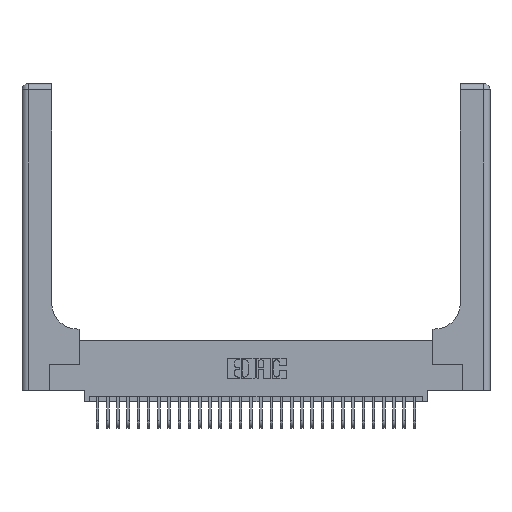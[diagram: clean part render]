
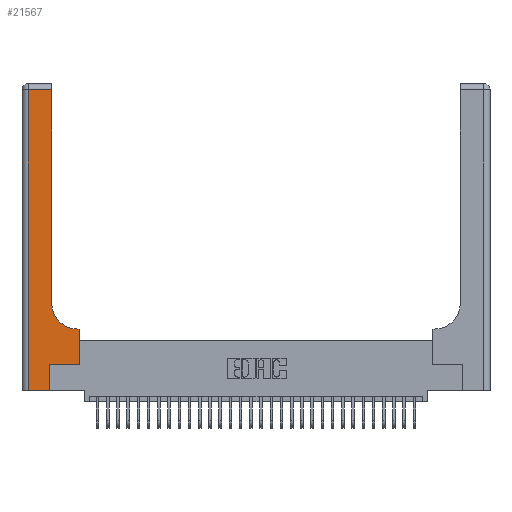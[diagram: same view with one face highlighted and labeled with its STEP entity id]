
A CAD part, top view. The second image highlights one B-rep face of the part: STEP entity #21567.
In plain terms, the highlighted planar face has unit normal (0, 0, 1).
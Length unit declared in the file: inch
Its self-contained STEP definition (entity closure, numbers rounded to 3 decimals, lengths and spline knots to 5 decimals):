
#291 = ORIENTED_EDGE ( 'NONE', *, *, #17191, .T. ) ;
#525 = CARTESIAN_POINT ( 'NONE',  ( 0.5585, 0.25, 0.37 ) ) ;
#1414 = FACE_OUTER_BOUND ( 'NONE', #19779, .T. ) ;
#1512 = CARTESIAN_POINT ( 'NONE',  ( 0.269, 0.25, 0.37 ) ) ;
#2704 = CARTESIAN_POINT ( 'NONE',  ( 0.5585, 0.6, 0.37 ) ) ;
#3283 = LINE ( 'NONE', #10654, #8548 ) ;
#3613 = EDGE_CURVE ( 'NONE', #7267, #27339, #28701, .T. ) ;
#3993 = DIRECTION ( 'NONE',  ( -1., 0., 0. ) ) ;
#4004 = DIRECTION ( 'NONE',  ( 0., 1., 0. ) ) ;
#4543 = LINE ( 'NONE', #29493, #17528 ) ;
#4869 = CARTESIAN_POINT ( 'NONE',  ( 0.5415, 0.85, 0.37 ) ) ;
#5541 = VERTEX_POINT ( 'NONE', #20499 ) ;
#6205 = LINE ( 'NONE', #25804, #32009 ) ;
#7267 = VERTEX_POINT ( 'NONE', #17939 ) ;
#7470 = DIRECTION ( 'NONE',  ( 1., 0., 0. ) ) ;
#7866 = CARTESIAN_POINT ( 'NONE',  ( 0.06, 2.94, 0.37 ) ) ;
#8024 = PLANE ( 'NONE',  #22975 ) ;
#8548 = VECTOR ( 'NONE', #33169, 39.37008 ) ;
#8583 = VERTEX_POINT ( 'NONE', #23969 ) ;
#9338 = VERTEX_POINT ( 'NONE', #1512 ) ;
#9535 = LINE ( 'NONE', #29439, #30106 ) ;
#10598 = CIRCLE ( 'NONE', #12292, 0.25 ) ;
#10619 = CARTESIAN_POINT ( 'NONE',  ( 0., 3., 0.37 ) ) ;
#10654 = CARTESIAN_POINT ( 'NONE',  ( 0.269, 0., 0.37 ) ) ;
#12292 = AXIS2_PLACEMENT_3D ( 'NONE', #4869, #22955, #7470 ) ;
#12900 = DIRECTION ( 'NONE',  ( 0., -1., 0. ) ) ;
#13208 = VERTEX_POINT ( 'NONE', #7866 ) ;
#13221 = DIRECTION ( 'NONE',  ( -1., 0., 0. ) ) ;
#13995 = DIRECTION ( 'NONE',  ( 1., 0., 0. ) ) ;
#14160 = CARTESIAN_POINT ( 'NONE',  ( 0.5415, 0.6, 0.37 ) ) ;
#14163 = VECTOR ( 'NONE', #4004, 39.37008 ) ;
#14220 = CARTESIAN_POINT ( 'NONE',  ( 0.269, 0.25, 0.37 ) ) ;
#14276 = LINE ( 'NONE', #525, #28006 ) ;
#14910 = LINE ( 'NONE', #19503, #27798 ) ;
#17191 = EDGE_CURVE ( 'NONE', #9338, #5541, #29421, .T. ) ;
#17528 = VECTOR ( 'NONE', #32068, 39.37008 ) ;
#17809 = ORIENTED_EDGE ( 'NONE', *, *, #25847, .T. ) ;
#17835 = VERTEX_POINT ( 'NONE', #30077 ) ;
#17939 = CARTESIAN_POINT ( 'NONE',  ( 0.2915, 0.85, 0.37 ) ) ;
#19503 = CARTESIAN_POINT ( 'NONE',  ( 0., 2.94, 0.37 ) ) ;
#19715 = ORIENTED_EDGE ( 'NONE', *, *, #24186, .T. ) ;
#19779 = EDGE_LOOP ( 'NONE', ( #20834, #30894, #25755, #32157, #19715, #291, #21763, #31819, #17809 ) ) ;
#20499 = CARTESIAN_POINT ( 'NONE',  ( 0.5585, 0.25, 0.37 ) ) ;
#20834 = ORIENTED_EDGE ( 'NONE', *, *, #3613, .T. ) ;
#21060 = VERTEX_POINT ( 'NONE', #2704 ) ;
#21232 = DIRECTION ( 'NONE',  ( 0., 1., 0. ) ) ;
#21567 = ADVANCED_FACE ( 'NONE', ( #1414 ), #8024, .F. ) ;
#21763 = ORIENTED_EDGE ( 'NONE', *, *, #31767, .T. ) ;
#21778 = EDGE_CURVE ( 'NONE', #17835, #8583, #9535, .T. ) ;
#21905 = DIRECTION ( 'NONE',  ( 1., 0., 0. ) ) ;
#22585 = VECTOR ( 'NONE', #21905, 39.37008 ) ;
#22955 = DIRECTION ( 'NONE',  ( 0., 0., -1. ) ) ;
#22975 = AXIS2_PLACEMENT_3D ( 'NONE', #10619, #28673, #13221 ) ;
#23845 = EDGE_CURVE ( 'NONE', #21060, #31265, #4543, .T. ) ;
#23969 = CARTESIAN_POINT ( 'NONE',  ( 0.269, 0., 0.37 ) ) ;
#24116 = CARTESIAN_POINT ( 'NONE',  ( 0.2915, 2.94, 0.37 ) ) ;
#24186 = EDGE_CURVE ( 'NONE', #8583, #9338, #3283, .T. ) ;
#25755 = ORIENTED_EDGE ( 'NONE', *, *, #31593, .T. ) ;
#25804 = CARTESIAN_POINT ( 'NONE',  ( 0.06, 3., 0.37 ) ) ;
#25847 = EDGE_CURVE ( 'NONE', #31265, #7267, #10598, .T. ) ;
#27339 = VERTEX_POINT ( 'NONE', #24116 ) ;
#27798 = VECTOR ( 'NONE', #3993, 39.37008 ) ;
#28006 = VECTOR ( 'NONE', #21232, 39.37008 ) ;
#28194 = EDGE_CURVE ( 'NONE', #27339, #13208, #14910, .T. ) ;
#28673 = DIRECTION ( 'NONE',  ( 0., 0., -1. ) ) ;
#28701 = LINE ( 'NONE', #32318, #14163 ) ;
#29421 = LINE ( 'NONE', #14220, #22585 ) ;
#29439 = CARTESIAN_POINT ( 'NONE',  ( 0., 0., 0.37 ) ) ;
#29493 = CARTESIAN_POINT ( 'NONE',  ( 0.2915, 0.6, 0.37 ) ) ;
#30077 = CARTESIAN_POINT ( 'NONE',  ( 0.06, 0., 0.37 ) ) ;
#30106 = VECTOR ( 'NONE', #13995, 39.37008 ) ;
#30894 = ORIENTED_EDGE ( 'NONE', *, *, #28194, .T. ) ;
#31265 = VERTEX_POINT ( 'NONE', #14160 ) ;
#31593 = EDGE_CURVE ( 'NONE', #13208, #17835, #6205, .T. ) ;
#31767 = EDGE_CURVE ( 'NONE', #5541, #21060, #14276, .T. ) ;
#31819 = ORIENTED_EDGE ( 'NONE', *, *, #23845, .T. ) ;
#32009 = VECTOR ( 'NONE', #12900, 39.37008 ) ;
#32068 = DIRECTION ( 'NONE',  ( -1., 0., 0. ) ) ;
#32157 = ORIENTED_EDGE ( 'NONE', *, *, #21778, .T. ) ;
#32318 = CARTESIAN_POINT ( 'NONE',  ( 0.2915, 3., 0.37 ) ) ;
#33169 = DIRECTION ( 'NONE',  ( 0., 1., 0. ) ) ;
